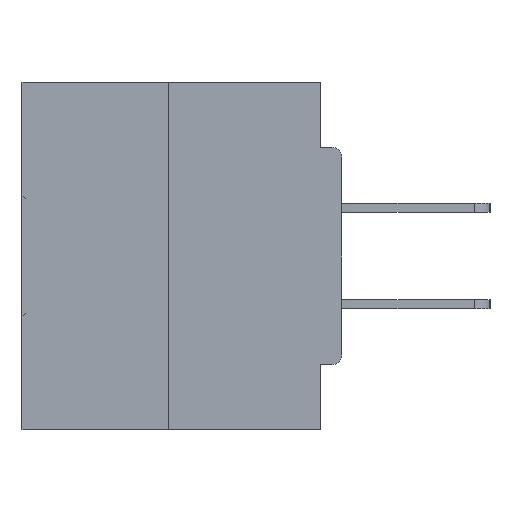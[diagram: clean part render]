
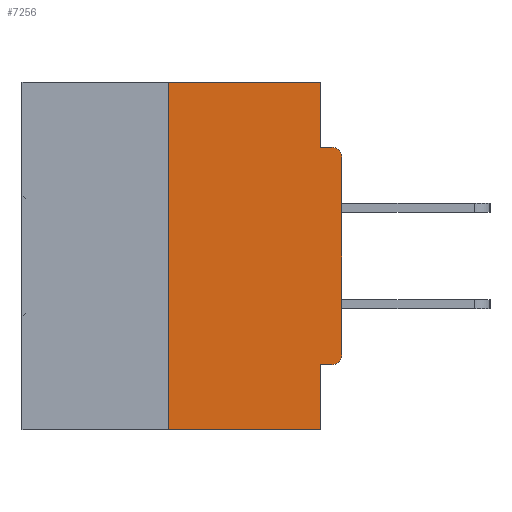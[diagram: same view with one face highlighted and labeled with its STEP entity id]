
A CAD part, left-side view. The second image highlights one B-rep face of the part: STEP entity #7256.
In plain terms, the highlighted planar face has unit normal (-1, 0, 0).
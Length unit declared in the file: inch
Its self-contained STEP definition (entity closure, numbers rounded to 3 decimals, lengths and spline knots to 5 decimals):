
#1515 = DIRECTION ( 'NONE',  ( 0., 0., -1. ) ) ;
#1684 = CARTESIAN_POINT ( 'NONE',  ( 0., 0., -0.3915 ) ) ;
#1781 = DIRECTION ( 'NONE',  ( 1., 0., 0. ) ) ;
#2921 = EDGE_CURVE ( 'NONE', #6822, #27200, #17224, .T. ) ;
#3574 = VERTEX_POINT ( 'NONE', #40349 ) ;
#4247 = CARTESIAN_POINT ( 'NONE',  ( 0., 0.015, -0.3915 ) ) ;
#4304 = DIRECTION ( 'NONE',  ( 0., 0., 1. ) ) ;
#4385 = CARTESIAN_POINT ( 'NONE',  ( 0., 0.46, 0. ) ) ;
#4568 = EDGE_LOOP ( 'NONE', ( #32076, #31039, #12381, #13664, #38217, #41577, #8428, #30459, #37264, #17271 ) ) ;
#4827 = FACE_OUTER_BOUND ( 'NONE', #4568, .T. ) ;
#5549 = CARTESIAN_POINT ( 'NONE',  ( 0., 0.031, -0.0935 ) ) ;
#6342 = CARTESIAN_POINT ( 'NONE',  ( 0., 0., -0.1085 ) ) ;
#6654 = LINE ( 'NONE', #23395, #26104 ) ;
#6822 = VERTEX_POINT ( 'NONE', #41564 ) ;
#6855 = CIRCLE ( 'NONE', #29777, 0.015 ) ;
#7058 = DIRECTION ( 'NONE',  ( 0., -1., 0. ) ) ;
#7256 = ADVANCED_FACE ( 'NONE', ( #4827 ), #10926, .F. ) ;
#8428 = ORIENTED_EDGE ( 'NONE', *, *, #33279, .T. ) ;
#8584 = LINE ( 'NONE', #41797, #20668 ) ;
#8806 = DIRECTION ( 'NONE',  ( 0., 0., 1. ) ) ;
#9024 = VERTEX_POINT ( 'NONE', #5549 ) ;
#9262 = CARTESIAN_POINT ( 'NONE',  ( 0., 0.031, -0.5 ) ) ;
#9434 = CARTESIAN_POINT ( 'NONE',  ( 0., 0.015, -0.0935 ) ) ;
#10926 = PLANE ( 'NONE',  #27642 ) ;
#10993 = DIRECTION ( 'NONE',  ( -1., 0., 0. ) ) ;
#11452 = LINE ( 'NONE', #24712, #24148 ) ;
#11476 = VECTOR ( 'NONE', #11987, 39.37008 ) ;
#11987 = DIRECTION ( 'NONE',  ( 0., 0., -1. ) ) ;
#12381 = ORIENTED_EDGE ( 'NONE', *, *, #2921, .T. ) ;
#13664 = ORIENTED_EDGE ( 'NONE', *, *, #18870, .F. ) ;
#14191 = LINE ( 'NONE', #20304, #28209 ) ;
#16236 = CARTESIAN_POINT ( 'NONE',  ( 0., 0.015, -0.1085 ) ) ;
#17160 = LINE ( 'NONE', #31271, #36529 ) ;
#17224 = LINE ( 'NONE', #23944, #42753 ) ;
#17271 = ORIENTED_EDGE ( 'NONE', *, *, #24349, .F. ) ;
#17563 = CARTESIAN_POINT ( 'NONE',  ( 0., 0., -0.0935 ) ) ;
#17995 = CIRCLE ( 'NONE', #25657, 0.015 ) ;
#18206 = LINE ( 'NONE', #17563, #28891 ) ;
#18870 = EDGE_CURVE ( 'NONE', #34635, #27200, #17160, .T. ) ;
#20304 = CARTESIAN_POINT ( 'NONE',  ( 0., 0.46, 0. ) ) ;
#20668 = VECTOR ( 'NONE', #8806, 39.37008 ) ;
#22241 = VERTEX_POINT ( 'NONE', #1684 ) ;
#22533 = EDGE_CURVE ( 'NONE', #27875, #22241, #6855, .T. ) ;
#22773 = DIRECTION ( 'NONE',  ( 0., 0., -1. ) ) ;
#22862 = VERTEX_POINT ( 'NONE', #9434 ) ;
#23395 = CARTESIAN_POINT ( 'NONE',  ( 0., 0., -0.4065 ) ) ;
#23648 = EDGE_CURVE ( 'NONE', #27875, #34635, #6654, .T. ) ;
#23944 = CARTESIAN_POINT ( 'NONE',  ( 0., 0.46, -0.5 ) ) ;
#24148 = VECTOR ( 'NONE', #4304, 39.37008 ) ;
#24349 = EDGE_CURVE ( 'NONE', #34213, #9024, #41736, .T. ) ;
#24389 = DIRECTION ( 'NONE',  ( 0., -1., 0. ) ) ;
#24712 = CARTESIAN_POINT ( 'NONE',  ( 0., 0.25, 0. ) ) ;
#24808 = DIRECTION ( 'NONE',  ( 0., 0., -1. ) ) ;
#25298 = EDGE_CURVE ( 'NONE', #9024, #22862, #18206, .T. ) ;
#25657 = AXIS2_PLACEMENT_3D ( 'NONE', #16236, #39482, #22773 ) ;
#26104 = VECTOR ( 'NONE', #29073, 39.37008 ) ;
#27200 = VERTEX_POINT ( 'NONE', #9262 ) ;
#27591 = DIRECTION ( 'NONE',  ( 0., -1., 0. ) ) ;
#27642 = AXIS2_PLACEMENT_3D ( 'NONE', #4385, #1781, #24808 ) ;
#27875 = VERTEX_POINT ( 'NONE', #33939 ) ;
#28209 = VECTOR ( 'NONE', #7058, 39.37008 ) ;
#28891 = VECTOR ( 'NONE', #27591, 39.37008 ) ;
#29073 = DIRECTION ( 'NONE',  ( 0., 1., 0. ) ) ;
#29233 = CARTESIAN_POINT ( 'NONE',  ( 0., 0.031, -0.4065 ) ) ;
#29488 = CARTESIAN_POINT ( 'NONE',  ( 0., 0.031, 0. ) ) ;
#29777 = AXIS2_PLACEMENT_3D ( 'NONE', #4247, #10993, #37458 ) ;
#30459 = ORIENTED_EDGE ( 'NONE', *, *, #41153, .T. ) ;
#31039 = ORIENTED_EDGE ( 'NONE', *, *, #39590, .F. ) ;
#31271 = CARTESIAN_POINT ( 'NONE',  ( 0., 0.031, -0.5 ) ) ;
#32076 = ORIENTED_EDGE ( 'NONE', *, *, #36057, .F. ) ;
#33279 = EDGE_CURVE ( 'NONE', #22241, #40721, #8584, .T. ) ;
#33939 = CARTESIAN_POINT ( 'NONE',  ( 0., 0.015, -0.4065 ) ) ;
#34213 = VERTEX_POINT ( 'NONE', #29488 ) ;
#34635 = VERTEX_POINT ( 'NONE', #29233 ) ;
#34788 = CARTESIAN_POINT ( 'NONE',  ( 0., 0.031, 0. ) ) ;
#36057 = EDGE_CURVE ( 'NONE', #3574, #34213, #14191, .T. ) ;
#36529 = VECTOR ( 'NONE', #1515, 39.37008 ) ;
#37264 = ORIENTED_EDGE ( 'NONE', *, *, #25298, .F. ) ;
#37458 = DIRECTION ( 'NONE',  ( 0., 0., -1. ) ) ;
#38217 = ORIENTED_EDGE ( 'NONE', *, *, #23648, .F. ) ;
#39482 = DIRECTION ( 'NONE',  ( -1., 0., 0. ) ) ;
#39590 = EDGE_CURVE ( 'NONE', #6822, #3574, #11452, .T. ) ;
#40349 = CARTESIAN_POINT ( 'NONE',  ( 0., 0.25, 0. ) ) ;
#40721 = VERTEX_POINT ( 'NONE', #6342 ) ;
#41153 = EDGE_CURVE ( 'NONE', #40721, #22862, #17995, .T. ) ;
#41564 = CARTESIAN_POINT ( 'NONE',  ( 0., 0.25, -0.5 ) ) ;
#41577 = ORIENTED_EDGE ( 'NONE', *, *, #22533, .T. ) ;
#41736 = LINE ( 'NONE', #34788, #11476 ) ;
#41797 = CARTESIAN_POINT ( 'NONE',  ( 0., 0., 0. ) ) ;
#42753 = VECTOR ( 'NONE', #24389, 39.37008 ) ;
